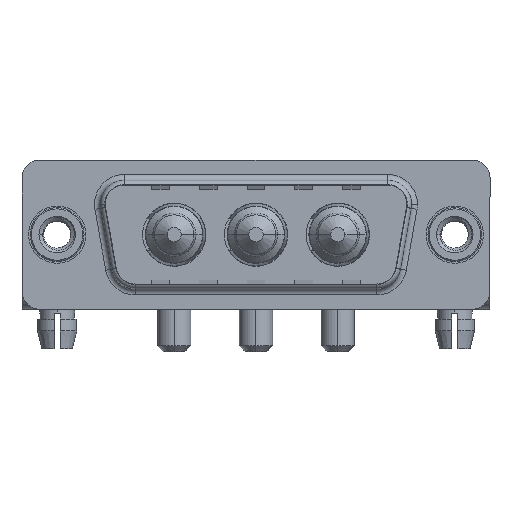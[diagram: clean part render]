
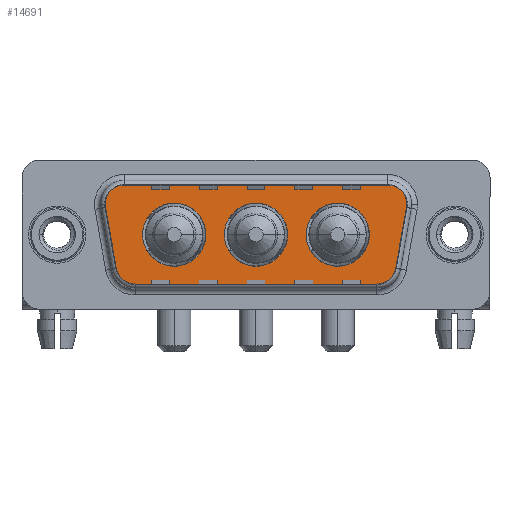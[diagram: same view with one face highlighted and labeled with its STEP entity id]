
A CAD part, top view. The second image highlights one B-rep face of the part: STEP entity #14691.
In plain terms, the highlighted planar face has unit normal (0, 0, 1).
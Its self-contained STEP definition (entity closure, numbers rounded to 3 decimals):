
#146 = CARTESIAN_POINT ( 'NONE',  ( 29.859, 2.553, 0. ) ) ;
#181 = VERTEX_POINT ( 'NONE', #5395 ) ;
#262 = DIRECTION ( 'NONE',  ( 0., 0., 1. ) ) ;
#273 = VERTEX_POINT ( 'NONE', #12856 ) ;
#361 = ORIENTED_EDGE ( 'NONE', *, *, #10980, .T. ) ;
#378 = CARTESIAN_POINT ( 'NONE',  ( 27.889, 4.9, 0. ) ) ;
#504 = CARTESIAN_POINT ( 'NONE',  ( 28.836, -3.247, 0. ) ) ;
#733 = AXIS2_PLACEMENT_3D ( 'NONE', #4863, #12572, #1188 ) ;
#817 = PLANE ( 'NONE',  #1305 ) ;
#836 = CARTESIAN_POINT ( 'NONE',  ( 19.3, 0., 0. ) ) ;
#869 = DIRECTION ( 'NONE',  ( -1., 0., 0. ) ) ;
#871 = EDGE_CURVE ( 'NONE', #273, #10255, #12891, .T. ) ;
#893 = CIRCLE ( 'NONE', #3023, 2.65 ) ;
#995 = CARTESIAN_POINT ( 'NONE',  ( 9.8, 0., 0. ) ) ;
#1149 = ORIENTED_EDGE ( 'NONE', *, *, #2019, .T. ) ;
#1188 = DIRECTION ( 'NONE',  ( -1., 0., 0. ) ) ;
#1205 = DIRECTION ( 'NONE',  ( 1., 0., 0. ) ) ;
#1305 = AXIS2_PLACEMENT_3D ( 'NONE', #5902, #2156, #14935 ) ;
#1444 = CARTESIAN_POINT ( 'NONE',  ( 23.5, 0., 0. ) ) ;
#1506 = VERTEX_POINT ( 'NONE', #4998 ) ;
#1610 = EDGE_CURVE ( 'NONE', #7875, #1769, #9518, .T. ) ;
#1650 = DIRECTION ( 'NONE',  ( 0., 0., 1. ) ) ;
#1769 = VERTEX_POINT ( 'NONE', #378 ) ;
#1781 = CIRCLE ( 'NONE', #3111, 2.65 ) ;
#1942 = CIRCLE ( 'NONE', #8819, 2.65 ) ;
#1997 = VECTOR ( 'NONE', #10905, 1000. ) ;
#2019 = EDGE_CURVE ( 'NONE', #1769, #181, #15999, .T. ) ;
#2156 = DIRECTION ( 'NONE',  ( 0., 0., 1. ) ) ;
#2161 = VERTEX_POINT ( 'NONE', #8754 ) ;
#2317 = DIRECTION ( 'NONE',  ( 0., 0., 1. ) ) ;
#2320 = AXIS2_PLACEMENT_3D ( 'NONE', #13025, #1650, #6733 ) ;
#2520 = CARTESIAN_POINT ( 'NONE',  ( 29.889, 2.9, 0. ) ) ;
#2800 = EDGE_CURVE ( 'NONE', #15507, #2161, #1942, .T. ) ;
#3023 = AXIS2_PLACEMENT_3D ( 'NONE', #8678, #12587, #1205 ) ;
#3085 = AXIS2_PLACEMENT_3D ( 'NONE', #7939, #4211, #6951 ) ;
#3111 = AXIS2_PLACEMENT_3D ( 'NONE', #1444, #14814, #7017 ) ;
#3237 = FACE_BOUND ( 'NONE', #11121, .T. ) ;
#3342 = EDGE_CURVE ( 'NONE', #11777, #6762, #893, .T. ) ;
#3412 = VERTEX_POINT ( 'NONE', #11177 ) ;
#3487 = DIRECTION ( 'NONE',  ( 0., 0., 1. ) ) ;
#3767 = EDGE_CURVE ( 'NONE', #4809, #13822, #13643, .T. ) ;
#4060 = ORIENTED_EDGE ( 'NONE', *, *, #7539, .F. ) ;
#4211 = DIRECTION ( 'NONE',  ( 0., 0., 1. ) ) ;
#4240 = ORIENTED_EDGE ( 'NONE', *, *, #11538, .T. ) ;
#4245 = VECTOR ( 'NONE', #5206, 1000. ) ;
#4423 = CARTESIAN_POINT ( 'NONE',  ( 9.8, 0., 0. ) ) ;
#4474 = CARTESIAN_POINT ( 'NONE',  ( 26.15, 0., 0. ) ) ;
#4487 = AXIS2_PLACEMENT_3D ( 'NONE', #14848, #3487, #6142 ) ;
#4493 = CARTESIAN_POINT ( 'NONE',  ( 3.441, 2.553, 0. ) ) ;
#4809 = VERTEX_POINT ( 'NONE', #4493 ) ;
#4863 = CARTESIAN_POINT ( 'NONE',  ( 6.434, -2.9, 0. ) ) ;
#4998 = CARTESIAN_POINT ( 'NONE',  ( 29.859, 2.553, 0. ) ) ;
#5128 = LINE ( 'NONE', #10500, #4245 ) ;
#5206 = DIRECTION ( 'NONE',  ( 1., 0., 0. ) ) ;
#5220 = DIRECTION ( 'NONE',  ( 0.174, 0.985, 0. ) ) ;
#5296 = VERTEX_POINT ( 'NONE', #15229 ) ;
#5342 = DIRECTION ( 'NONE',  ( 1., 0., 0. ) ) ;
#5395 = CARTESIAN_POINT ( 'NONE',  ( 5.411, 4.9, 0. ) ) ;
#5481 = VECTOR ( 'NONE', #5220, 1000. ) ;
#5902 = CARTESIAN_POINT ( 'NONE',  ( 26.866, -2.9, 0. ) ) ;
#5995 = DIRECTION ( 'NONE',  ( 0., 0., 1. ) ) ;
#6055 = CARTESIAN_POINT ( 'NONE',  ( 14., 0., 0. ) ) ;
#6142 = DIRECTION ( 'NONE',  ( -1., 0., 0. ) ) ;
#6395 = ORIENTED_EDGE ( 'NONE', *, *, #11269, .F. ) ;
#6733 = DIRECTION ( 'NONE',  ( 1., 0., 0. ) ) ;
#6762 = VERTEX_POINT ( 'NONE', #6055 ) ;
#6778 = DIRECTION ( 'NONE',  ( 1., 0., 0. ) ) ;
#6928 = VECTOR ( 'NONE', #869, 1000. ) ;
#6951 = DIRECTION ( 'NONE',  ( 1., 0., 0. ) ) ;
#7017 = DIRECTION ( 'NONE',  ( 1., 0., 0. ) ) ;
#7318 = EDGE_LOOP ( 'NONE', ( #11133, #8322, #361, #8245, #1149, #13232, #16376, #4240, #11596 ) ) ;
#7389 = EDGE_LOOP ( 'NONE', ( #15660, #13621 ) ) ;
#7460 = DIRECTION ( 'NONE',  ( 1., 0., 0. ) ) ;
#7539 = EDGE_CURVE ( 'NONE', #2161, #15507, #13656, .T. ) ;
#7615 = AXIS2_PLACEMENT_3D ( 'NONE', #7767, #9096, #6778 ) ;
#7767 = CARTESIAN_POINT ( 'NONE',  ( 23.5, 0., 0. ) ) ;
#7827 = AXIS2_PLACEMENT_3D ( 'NONE', #995, #5995, #16034 ) ;
#7875 = VERTEX_POINT ( 'NONE', #2520 ) ;
#7889 = CIRCLE ( 'NONE', #14228, 2. ) ;
#7939 = CARTESIAN_POINT ( 'NONE',  ( 26.866, -2.9, 0. ) ) ;
#8082 = CARTESIAN_POINT ( 'NONE',  ( 4.464, -3.247, 0. ) ) ;
#8245 = ORIENTED_EDGE ( 'NONE', *, *, #1610, .T. ) ;
#8296 = FACE_BOUND ( 'NONE', #10321, .T. ) ;
#8322 = ORIENTED_EDGE ( 'NONE', *, *, #10142, .T. ) ;
#8336 = CARTESIAN_POINT ( 'NONE',  ( 12.45, 0., 0. ) ) ;
#8375 = FACE_BOUND ( 'NONE', #7389, .T. ) ;
#8675 = CARTESIAN_POINT ( 'NONE',  ( 5.411, 4.9, 0. ) ) ;
#8678 = CARTESIAN_POINT ( 'NONE',  ( 16.65, 0., 0. ) ) ;
#8692 = CARTESIAN_POINT ( 'NONE',  ( 5.411, 2.9, 0. ) ) ;
#8754 = CARTESIAN_POINT ( 'NONE',  ( 7.15, 0., 0. ) ) ;
#8796 = EDGE_CURVE ( 'NONE', #181, #4809, #12599, .T. ) ;
#8819 = AXIS2_PLACEMENT_3D ( 'NONE', #4423, #262, #5342 ) ;
#9096 = DIRECTION ( 'NONE',  ( 0., 0., 1. ) ) ;
#9518 = CIRCLE ( 'NONE', #4487, 2. ) ;
#9838 = ORIENTED_EDGE ( 'NONE', *, *, #2800, .F. ) ;
#10142 = EDGE_CURVE ( 'NONE', #10255, #1506, #12766, .T. ) ;
#10255 = VERTEX_POINT ( 'NONE', #504 ) ;
#10321 = EDGE_LOOP ( 'NONE', ( #9838, #4060 ) ) ;
#10500 = CARTESIAN_POINT ( 'NONE',  ( 6.434, -4.9, 0. ) ) ;
#10823 = EDGE_CURVE ( 'NONE', #6762, #11777, #15555, .T. ) ;
#10905 = DIRECTION ( 'NONE',  ( 0.174, -0.985, 0. ) ) ;
#10980 = EDGE_CURVE ( 'NONE', #1506, #7875, #7889, .T. ) ;
#11001 = AXIS2_PLACEMENT_3D ( 'NONE', #8692, #2317, #7460 ) ;
#11121 = EDGE_LOOP ( 'NONE', ( #16306, #6395 ) ) ;
#11133 = ORIENTED_EDGE ( 'NONE', *, *, #871, .T. ) ;
#11177 = CARTESIAN_POINT ( 'NONE',  ( 6.434, -4.9, 0. ) ) ;
#11226 = EDGE_CURVE ( 'NONE', #16427, #5296, #14506, .T. ) ;
#11269 = EDGE_CURVE ( 'NONE', #5296, #16427, #1781, .T. ) ;
#11538 = EDGE_CURVE ( 'NONE', #13822, #3412, #15064, .T. ) ;
#11596 = ORIENTED_EDGE ( 'NONE', *, *, #15341, .T. ) ;
#11749 = DIRECTION ( 'NONE',  ( -1., 0., 0. ) ) ;
#11777 = VERTEX_POINT ( 'NONE', #836 ) ;
#12280 = FACE_OUTER_BOUND ( 'NONE', #7318, .T. ) ;
#12572 = DIRECTION ( 'NONE',  ( 0., 0., 1. ) ) ;
#12587 = DIRECTION ( 'NONE',  ( 0., 0., 1. ) ) ;
#12599 = CIRCLE ( 'NONE', #11001, 2. ) ;
#12766 = LINE ( 'NONE', #146, #5481 ) ;
#12856 = CARTESIAN_POINT ( 'NONE',  ( 26.866, -4.9, 0. ) ) ;
#12891 = CIRCLE ( 'NONE', #3085, 2. ) ;
#13025 = CARTESIAN_POINT ( 'NONE',  ( 16.65, 0., 0. ) ) ;
#13232 = ORIENTED_EDGE ( 'NONE', *, *, #8796, .T. ) ;
#13621 = ORIENTED_EDGE ( 'NONE', *, *, #10823, .F. ) ;
#13643 = LINE ( 'NONE', #14896, #1997 ) ;
#13656 = CIRCLE ( 'NONE', #7827, 2.65 ) ;
#13822 = VERTEX_POINT ( 'NONE', #8082 ) ;
#14228 = AXIS2_PLACEMENT_3D ( 'NONE', #14319, #15491, #11749 ) ;
#14319 = CARTESIAN_POINT ( 'NONE',  ( 27.889, 2.9, 0. ) ) ;
#14506 = CIRCLE ( 'NONE', #7615, 2.65 ) ;
#14691 = ADVANCED_FACE ( 'NONE', ( #8375, #3237, #8296, #12280 ), #817, .T. ) ;
#14814 = DIRECTION ( 'NONE',  ( 0., 0., 1. ) ) ;
#14848 = CARTESIAN_POINT ( 'NONE',  ( 27.889, 2.9, 0. ) ) ;
#14896 = CARTESIAN_POINT ( 'NONE',  ( 3.441, 2.553, 0. ) ) ;
#14935 = DIRECTION ( 'NONE',  ( 1., 0., 0. ) ) ;
#15064 = CIRCLE ( 'NONE', #733, 2. ) ;
#15229 = CARTESIAN_POINT ( 'NONE',  ( 20.85, 0., 0. ) ) ;
#15341 = EDGE_CURVE ( 'NONE', #3412, #273, #5128, .T. ) ;
#15491 = DIRECTION ( 'NONE',  ( 0., 0., 1. ) ) ;
#15507 = VERTEX_POINT ( 'NONE', #8336 ) ;
#15555 = CIRCLE ( 'NONE', #2320, 2.65 ) ;
#15660 = ORIENTED_EDGE ( 'NONE', *, *, #3342, .F. ) ;
#15999 = LINE ( 'NONE', #8675, #6928 ) ;
#16034 = DIRECTION ( 'NONE',  ( 1., 0., 0. ) ) ;
#16306 = ORIENTED_EDGE ( 'NONE', *, *, #11226, .F. ) ;
#16376 = ORIENTED_EDGE ( 'NONE', *, *, #3767, .T. ) ;
#16427 = VERTEX_POINT ( 'NONE', #4474 ) ;
